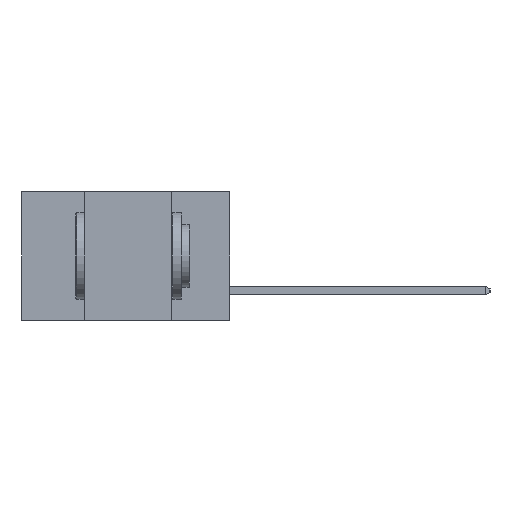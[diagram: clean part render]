
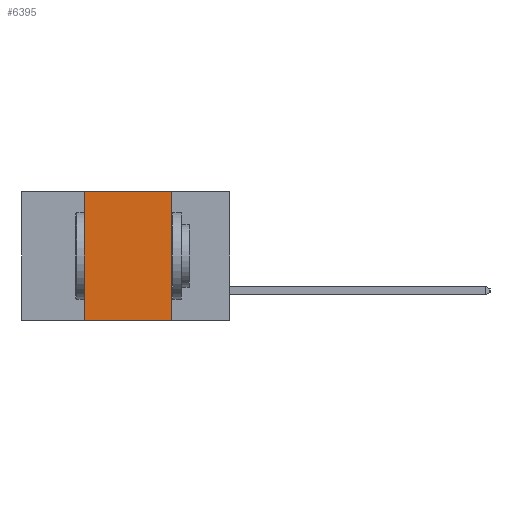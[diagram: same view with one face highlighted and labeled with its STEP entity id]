
A CAD part, left-side view. The second image highlights one B-rep face of the part: STEP entity #6395.
In plain terms, the highlighted planar face has unit normal (-1, 0, 0).
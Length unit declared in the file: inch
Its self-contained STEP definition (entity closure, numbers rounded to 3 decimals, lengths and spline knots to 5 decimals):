
#333 = CARTESIAN_POINT ( 'NONE',  ( 0., 0.17, -0.37 ) ) ;
#1185 = CARTESIAN_POINT ( 'NONE',  ( 0., 0.17, -0.37 ) ) ;
#1698 = CARTESIAN_POINT ( 'NONE',  ( 0., 0.6, 0. ) ) ;
#1812 = DIRECTION ( 'NONE',  ( 0., -1., 0. ) ) ;
#4062 = DIRECTION ( 'NONE',  ( 0., 0., -1. ) ) ;
#4704 = EDGE_CURVE ( 'NONE', #6019, #15620, #15050, .T. ) ;
#5110 = VECTOR ( 'NONE', #7337, 39.37008 ) ;
#5255 = DIRECTION ( 'NONE',  ( 0., 0., -1. ) ) ;
#5281 = DIRECTION ( 'NONE',  ( 1., 0., 0. ) ) ;
#5335 = CARTESIAN_POINT ( 'NONE',  ( 0., 0.6, 0. ) ) ;
#5371 = VERTEX_POINT ( 'NONE', #23245 ) ;
#5644 = PLANE ( 'NONE',  #22654 ) ;
#5660 = DIRECTION ( 'NONE',  ( 0., 0., 1. ) ) ;
#5705 = VERTEX_POINT ( 'NONE', #17658 ) ;
#6019 = VERTEX_POINT ( 'NONE', #12026 ) ;
#6395 = ADVANCED_FACE ( 'NONE', ( #18106 ), #5644, .F. ) ;
#6637 = EDGE_CURVE ( 'NONE', #5705, #5371, #23276, .T. ) ;
#6935 = CARTESIAN_POINT ( 'NONE',  ( 0., 0.6, -0.37 ) ) ;
#7337 = DIRECTION ( 'NONE',  ( 0., -1., 0. ) ) ;
#8916 = LINE ( 'NONE', #333, #23425 ) ;
#9499 = ORIENTED_EDGE ( 'NONE', *, *, #19169, .F. ) ;
#10890 = EDGE_LOOP ( 'NONE', ( #9499, #14824, #15413, #11575 ) ) ;
#11575 = ORIENTED_EDGE ( 'NONE', *, *, #4704, .T. ) ;
#12026 = CARTESIAN_POINT ( 'NONE',  ( 0., 0.42, -0.37 ) ) ;
#14824 = ORIENTED_EDGE ( 'NONE', *, *, #6637, .F. ) ;
#15050 = LINE ( 'NONE', #6935, #5110 ) ;
#15413 = ORIENTED_EDGE ( 'NONE', *, *, #17213, .F. ) ;
#15620 = VERTEX_POINT ( 'NONE', #1185 ) ;
#15790 = LINE ( 'NONE', #18696, #20588 ) ;
#17213 = EDGE_CURVE ( 'NONE', #6019, #5705, #15790, .T. ) ;
#17658 = CARTESIAN_POINT ( 'NONE',  ( 0., 0.42, 0. ) ) ;
#18106 = FACE_OUTER_BOUND ( 'NONE', #10890, .T. ) ;
#18696 = CARTESIAN_POINT ( 'NONE',  ( 0., 0.42, -0.37 ) ) ;
#19169 = EDGE_CURVE ( 'NONE', #5371, #15620, #8916, .T. ) ;
#20588 = VECTOR ( 'NONE', #5660, 39.37008 ) ;
#22227 = VECTOR ( 'NONE', #1812, 39.37008 ) ;
#22654 = AXIS2_PLACEMENT_3D ( 'NONE', #5335, #5281, #5255 ) ;
#23245 = CARTESIAN_POINT ( 'NONE',  ( 0., 0.17, 0. ) ) ;
#23276 = LINE ( 'NONE', #1698, #22227 ) ;
#23425 = VECTOR ( 'NONE', #4062, 39.37008 ) ;
